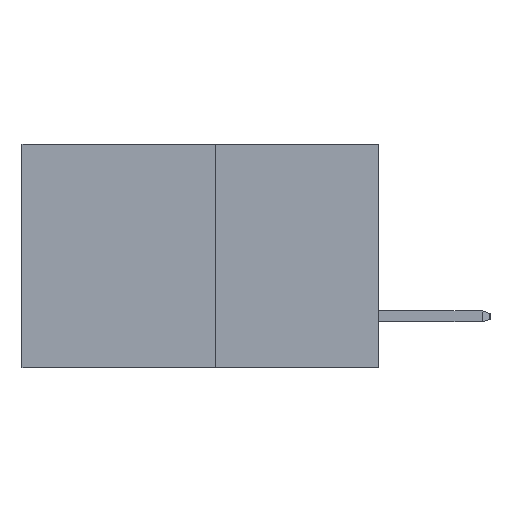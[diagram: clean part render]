
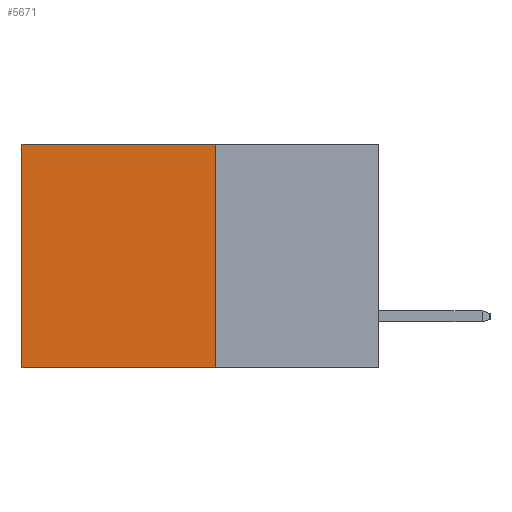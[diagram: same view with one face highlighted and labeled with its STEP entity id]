
A CAD part, left-side view. The second image highlights one B-rep face of the part: STEP entity #5671.
In plain terms, the highlighted planar face has unit normal (-1, 0, 0).
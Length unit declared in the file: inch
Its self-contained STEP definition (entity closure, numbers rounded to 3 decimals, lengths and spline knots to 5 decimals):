
#255 = VERTEX_POINT ( 'NONE', #12702 ) ;
#833 = VECTOR ( 'NONE', #10094, 39.37008 ) ;
#1918 = VERTEX_POINT ( 'NONE', #13377 ) ;
#2098 = ORIENTED_EDGE ( 'NONE', *, *, #21021, .T. ) ;
#5671 = ADVANCED_FACE ( 'NONE', ( #9793 ), #8015, .F. ) ;
#5814 = ORIENTED_EDGE ( 'NONE', *, *, #21695, .F. ) ;
#5832 = DIRECTION ( 'NONE',  ( 0., 1., 0. ) ) ;
#6212 = CARTESIAN_POINT ( 'NONE',  ( 0.277, 0.27, -0.37 ) ) ;
#6873 = CARTESIAN_POINT ( 'NONE',  ( 0.277, 0.27, -0.37 ) ) ;
#8015 = PLANE ( 'NONE',  #13719 ) ;
#8096 = LINE ( 'NONE', #9529, #17254 ) ;
#9529 = CARTESIAN_POINT ( 'NONE',  ( 0.277, 0.27, -0.37 ) ) ;
#9553 = LINE ( 'NONE', #18548, #18671 ) ;
#9663 = EDGE_CURVE ( 'NONE', #12502, #19395, #14096, .T. ) ;
#9793 = FACE_OUTER_BOUND ( 'NONE', #23329, .T. ) ;
#9852 = DIRECTION ( 'NONE',  ( 1., 0., 0. ) ) ;
#10094 = DIRECTION ( 'NONE',  ( 0., 0., -1. ) ) ;
#10279 = CARTESIAN_POINT ( 'NONE',  ( 0.277, 0.59, -0.37 ) ) ;
#10463 = LINE ( 'NONE', #11850, #833 ) ;
#11850 = CARTESIAN_POINT ( 'NONE',  ( 0.277, 0.59, -0.37 ) ) ;
#12502 = VERTEX_POINT ( 'NONE', #12923 ) ;
#12702 = CARTESIAN_POINT ( 'NONE',  ( 0.277, 0.59, 0. ) ) ;
#12923 = CARTESIAN_POINT ( 'NONE',  ( 0.277, 0.27, -0.37 ) ) ;
#13377 = CARTESIAN_POINT ( 'NONE',  ( 0.277, 0.27, 0. ) ) ;
#13719 = AXIS2_PLACEMENT_3D ( 'NONE', #6212, #9852, #22510 ) ;
#13973 = ORIENTED_EDGE ( 'NONE', *, *, #9663, .F. ) ;
#14096 = LINE ( 'NONE', #6873, #17752 ) ;
#14745 = EDGE_CURVE ( 'NONE', #255, #19395, #10463, .T. ) ;
#17254 = VECTOR ( 'NONE', #18601, 39.37008 ) ;
#17752 = VECTOR ( 'NONE', #23109, 39.37008 ) ;
#18548 = CARTESIAN_POINT ( 'NONE',  ( 0.277, 0.27, 0. ) ) ;
#18601 = DIRECTION ( 'NONE',  ( 0., 0., -1. ) ) ;
#18671 = VECTOR ( 'NONE', #5832, 39.37008 ) ;
#19395 = VERTEX_POINT ( 'NONE', #10279 ) ;
#21021 = EDGE_CURVE ( 'NONE', #1918, #255, #9553, .T. ) ;
#21695 = EDGE_CURVE ( 'NONE', #1918, #12502, #8096, .T. ) ;
#22510 = DIRECTION ( 'NONE',  ( 0., 0., -1. ) ) ;
#23109 = DIRECTION ( 'NONE',  ( 0., 1., 0. ) ) ;
#23155 = ORIENTED_EDGE ( 'NONE', *, *, #14745, .T. ) ;
#23329 = EDGE_LOOP ( 'NONE', ( #23155, #13973, #5814, #2098 ) ) ;
